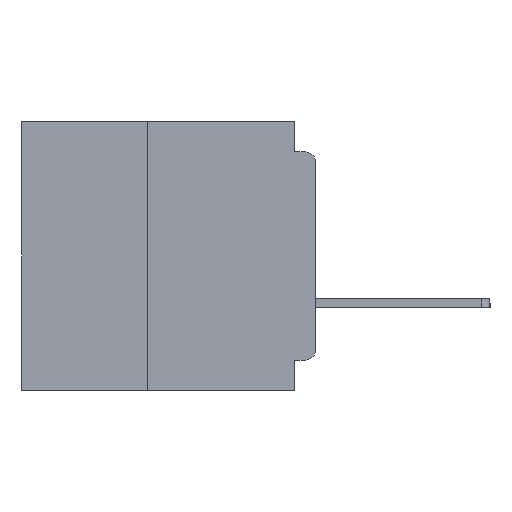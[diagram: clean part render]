
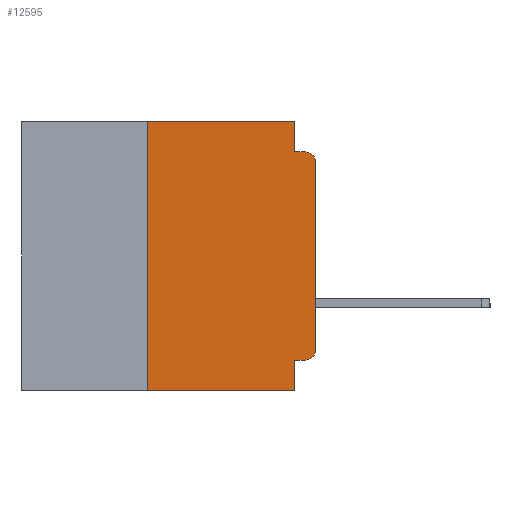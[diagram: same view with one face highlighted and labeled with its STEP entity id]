
A CAD part, left-side view. The second image highlights one B-rep face of the part: STEP entity #12595.
In plain terms, the highlighted planar face has unit normal (-1, 0, 0).
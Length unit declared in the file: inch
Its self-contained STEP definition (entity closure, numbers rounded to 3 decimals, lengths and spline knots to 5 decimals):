
#930 = ORIENTED_EDGE ( 'NONE', *, *, #13434, .F. ) ;
#1617 = VECTOR ( 'NONE', #24621, 39.37008 ) ;
#1910 = VERTEX_POINT ( 'NONE', #35689 ) ;
#1985 = VERTEX_POINT ( 'NONE', #9777 ) ;
#2051 = LINE ( 'NONE', #10083, #35294 ) ;
#2183 = DIRECTION ( 'NONE',  ( 0., 0., -1. ) ) ;
#2695 = FACE_OUTER_BOUND ( 'NONE', #7233, .T. ) ;
#3388 = CARTESIAN_POINT ( 'NONE',  ( 0., 0., -0.06 ) ) ;
#3929 = ORIENTED_EDGE ( 'NONE', *, *, #29719, .F. ) ;
#4287 = VERTEX_POINT ( 'NONE', #24712 ) ;
#4399 = VERTEX_POINT ( 'NONE', #21579 ) ;
#5369 = ORIENTED_EDGE ( 'NONE', *, *, #9534, .T. ) ;
#7233 = EDGE_LOOP ( 'NONE', ( #5369, #38564, #8357, #33251, #930, #3929, #37131, #21630, #31810, #26467 ) ) ;
#7254 = CIRCLE ( 'NONE', #24369, 0.015 ) ;
#7401 = VECTOR ( 'NONE', #34652, 39.37008 ) ;
#7512 = DIRECTION ( 'NONE',  ( 0., 0., 1. ) ) ;
#7758 = LINE ( 'NONE', #18129, #23435 ) ;
#8272 = CARTESIAN_POINT ( 'NONE',  ( 0., 0.031, -0.4 ) ) ;
#8357 = ORIENTED_EDGE ( 'NONE', *, *, #37453, .F. ) ;
#9245 = CIRCLE ( 'NONE', #26633, 0.015 ) ;
#9534 = EDGE_CURVE ( 'NONE', #35270, #35415, #36583, .T. ) ;
#9777 = CARTESIAN_POINT ( 'NONE',  ( 0., 0.031, -0.355 ) ) ;
#10083 = CARTESIAN_POINT ( 'NONE',  ( 0., 0.437, -0.4 ) ) ;
#10105 = VERTEX_POINT ( 'NONE', #16964 ) ;
#10196 = DIRECTION ( 'NONE',  ( 0., -1., 0. ) ) ;
#10313 = EDGE_CURVE ( 'NONE', #28977, #35270, #7254, .T. ) ;
#10606 = PLANE ( 'NONE',  #39491 ) ;
#12595 = ADVANCED_FACE ( 'NONE', ( #2695 ), #10606, .F. ) ;
#13434 = EDGE_CURVE ( 'NONE', #4399, #10105, #17418, .T. ) ;
#15085 = LINE ( 'NONE', #22657, #29667 ) ;
#15155 = DIRECTION ( 'NONE',  ( 0., 0., 1. ) ) ;
#15793 = LINE ( 'NONE', #33761, #39658 ) ;
#16660 = EDGE_CURVE ( 'NONE', #35415, #32839, #9245, .T. ) ;
#16952 = DIRECTION ( 'NONE',  ( 0., 0., -1. ) ) ;
#16964 = CARTESIAN_POINT ( 'NONE',  ( 0., 0.031, 0. ) ) ;
#17418 = LINE ( 'NONE', #27738, #1617 ) ;
#18085 = CARTESIAN_POINT ( 'NONE',  ( 0., 0.015, -0.06 ) ) ;
#18129 = CARTESIAN_POINT ( 'NONE',  ( 0., 0., -0.355 ) ) ;
#18545 = CARTESIAN_POINT ( 'NONE',  ( 0., 0.015, -0.045 ) ) ;
#20495 = VECTOR ( 'NONE', #34347, 39.37008 ) ;
#21016 = DIRECTION ( 'NONE',  ( -1., 0., 0. ) ) ;
#21215 = DIRECTION ( 'NONE',  ( 0., 0., -1. ) ) ;
#21257 = DIRECTION ( 'NONE',  ( 0., 1., 0. ) ) ;
#21414 = EDGE_CURVE ( 'NONE', #1985, #33892, #24049, .T. ) ;
#21579 = CARTESIAN_POINT ( 'NONE',  ( 0., 0.25, 0. ) ) ;
#21630 = ORIENTED_EDGE ( 'NONE', *, *, #21414, .F. ) ;
#22314 = CARTESIAN_POINT ( 'NONE',  ( 0., 0.031, -0.4 ) ) ;
#22657 = CARTESIAN_POINT ( 'NONE',  ( 0., 0., -0.045 ) ) ;
#22914 = EDGE_CURVE ( 'NONE', #28977, #1985, #7758, .T. ) ;
#22973 = CARTESIAN_POINT ( 'NONE',  ( 0., 0.015, -0.355 ) ) ;
#23435 = VECTOR ( 'NONE', #21257, 39.37008 ) ;
#24049 = LINE ( 'NONE', #22314, #7401 ) ;
#24369 = AXIS2_PLACEMENT_3D ( 'NONE', #39551, #21016, #2183 ) ;
#24515 = CARTESIAN_POINT ( 'NONE',  ( 0., 0., -0.34 ) ) ;
#24621 = DIRECTION ( 'NONE',  ( 0., -1., 0. ) ) ;
#24712 = CARTESIAN_POINT ( 'NONE',  ( 0., 0.25, -0.4 ) ) ;
#25544 = EDGE_CURVE ( 'NONE', #4287, #33892, #2051, .T. ) ;
#25647 = DIRECTION ( 'NONE',  ( 0., -1., 0. ) ) ;
#26467 = ORIENTED_EDGE ( 'NONE', *, *, #10313, .T. ) ;
#26490 = CARTESIAN_POINT ( 'NONE',  ( 0., 0., 0. ) ) ;
#26633 = AXIS2_PLACEMENT_3D ( 'NONE', #18085, #39736, #21215 ) ;
#27738 = CARTESIAN_POINT ( 'NONE',  ( 0., 0.437, 0. ) ) ;
#27752 = LINE ( 'NONE', #31231, #20495 ) ;
#28977 = VERTEX_POINT ( 'NONE', #22973 ) ;
#29317 = VECTOR ( 'NONE', #7512, 39.37008 ) ;
#29667 = VECTOR ( 'NONE', #10196, 39.37008 ) ;
#29719 = EDGE_CURVE ( 'NONE', #4287, #4399, #15793, .T. ) ;
#31231 = CARTESIAN_POINT ( 'NONE',  ( 0., 0.031, 0. ) ) ;
#31797 = EDGE_CURVE ( 'NONE', #10105, #1910, #27752, .T. ) ;
#31810 = ORIENTED_EDGE ( 'NONE', *, *, #22914, .F. ) ;
#32406 = CARTESIAN_POINT ( 'NONE',  ( 0., 0.437, 0. ) ) ;
#32839 = VERTEX_POINT ( 'NONE', #18545 ) ;
#33251 = ORIENTED_EDGE ( 'NONE', *, *, #31797, .F. ) ;
#33761 = CARTESIAN_POINT ( 'NONE',  ( 0., 0.25, -0.4 ) ) ;
#33892 = VERTEX_POINT ( 'NONE', #8272 ) ;
#34347 = DIRECTION ( 'NONE',  ( 0., 0., -1. ) ) ;
#34652 = DIRECTION ( 'NONE',  ( 0., 0., -1. ) ) ;
#35270 = VERTEX_POINT ( 'NONE', #24515 ) ;
#35294 = VECTOR ( 'NONE', #25647, 39.37008 ) ;
#35415 = VERTEX_POINT ( 'NONE', #3388 ) ;
#35513 = DIRECTION ( 'NONE',  ( 1., 0., 0. ) ) ;
#35689 = CARTESIAN_POINT ( 'NONE',  ( 0., 0.031, -0.045 ) ) ;
#36583 = LINE ( 'NONE', #26490, #29317 ) ;
#37131 = ORIENTED_EDGE ( 'NONE', *, *, #25544, .T. ) ;
#37453 = EDGE_CURVE ( 'NONE', #1910, #32839, #15085, .T. ) ;
#38564 = ORIENTED_EDGE ( 'NONE', *, *, #16660, .T. ) ;
#39491 = AXIS2_PLACEMENT_3D ( 'NONE', #32406, #35513, #16952 ) ;
#39551 = CARTESIAN_POINT ( 'NONE',  ( 0., 0.015, -0.34 ) ) ;
#39658 = VECTOR ( 'NONE', #15155, 39.37008 ) ;
#39736 = DIRECTION ( 'NONE',  ( -1., 0., 0. ) ) ;
